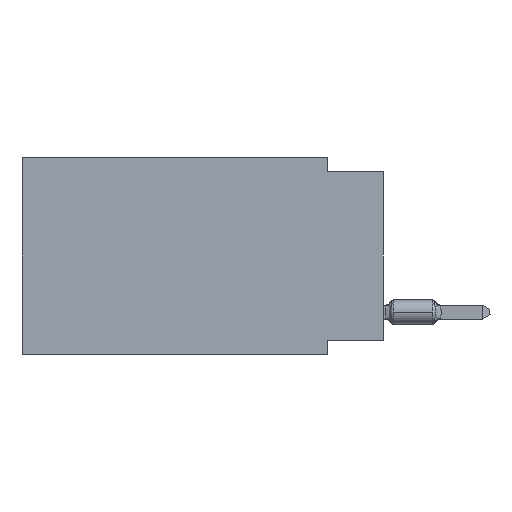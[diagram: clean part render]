
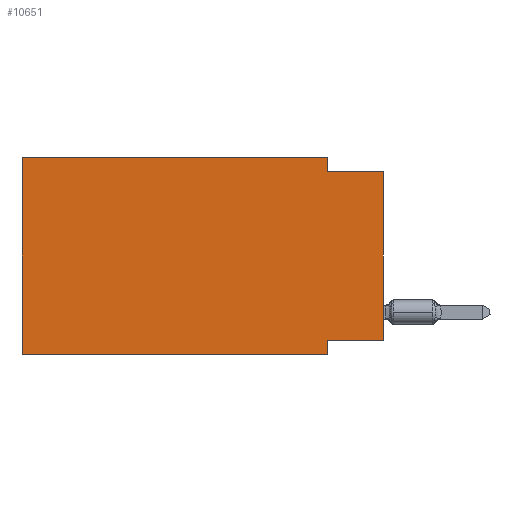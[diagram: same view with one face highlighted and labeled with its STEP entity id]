
A CAD part, left-side view. The second image highlights one B-rep face of the part: STEP entity #10651.
In plain terms, the highlighted planar face has unit normal (-1, 0, 0).
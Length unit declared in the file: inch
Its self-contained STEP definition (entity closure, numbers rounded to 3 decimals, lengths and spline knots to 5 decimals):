
#71 = VERTEX_POINT ( 'NONE', #4853 ) ;
#586 = VECTOR ( 'NONE', #7887, 39.37008 ) ;
#1035 = CARTESIAN_POINT ( 'NONE',  ( 0., 0., -0.025 ) ) ;
#1138 = VERTEX_POINT ( 'NONE', #14995 ) ;
#1370 = CARTESIAN_POINT ( 'NONE',  ( 0., 0.1, 0. ) ) ;
#1806 = LINE ( 'NONE', #6784, #7038 ) ;
#2073 = CARTESIAN_POINT ( 'NONE',  ( 0., 0., -0.325 ) ) ;
#2332 = CARTESIAN_POINT ( 'NONE',  ( 0., 0., 0. ) ) ;
#2393 = EDGE_CURVE ( 'NONE', #21580, #5204, #20155, .T. ) ;
#3198 = DIRECTION ( 'NONE',  ( 0., 0., -1. ) ) ;
#3773 = EDGE_LOOP ( 'NONE', ( #19470, #11132, #13963, #9775, #19159, #15180, #14685, #8173 ) ) ;
#4623 = LINE ( 'NONE', #13487, #4874 ) ;
#4830 = EDGE_CURVE ( 'NONE', #1138, #12046, #4623, .T. ) ;
#4840 = LINE ( 'NONE', #1035, #19109 ) ;
#4853 = CARTESIAN_POINT ( 'NONE',  ( 0., 0.1, -0.325 ) ) ;
#4874 = VECTOR ( 'NONE', #21982, 39.37008 ) ;
#5204 = VERTEX_POINT ( 'NONE', #16688 ) ;
#5229 = PLANE ( 'NONE',  #11575 ) ;
#5503 = EDGE_CURVE ( 'NONE', #12060, #8527, #16630, .T. ) ;
#6114 = LINE ( 'NONE', #13120, #12769 ) ;
#6492 = EDGE_CURVE ( 'NONE', #1138, #12060, #6114, .T. ) ;
#6784 = CARTESIAN_POINT ( 'NONE',  ( 0., 0.1, 0. ) ) ;
#7038 = VECTOR ( 'NONE', #3198, 39.37008 ) ;
#7044 = LINE ( 'NONE', #2073, #11892 ) ;
#7887 = DIRECTION ( 'NONE',  ( 0., -1., 0. ) ) ;
#7983 = DIRECTION ( 'NONE',  ( 0., 0., 1. ) ) ;
#8173 = ORIENTED_EDGE ( 'NONE', *, *, #16209, .F. ) ;
#8329 = CARTESIAN_POINT ( 'NONE',  ( 0., 0.1, -0.025 ) ) ;
#8519 = EDGE_CURVE ( 'NONE', #18264, #5204, #4840, .T. ) ;
#8527 = VERTEX_POINT ( 'NONE', #1370 ) ;
#8571 = DIRECTION ( 'NONE',  ( 0., 0., -1. ) ) ;
#8998 = DIRECTION ( 'NONE',  ( 0., 1., 0. ) ) ;
#9085 = CARTESIAN_POINT ( 'NONE',  ( 0., 0., -0.325 ) ) ;
#9775 = ORIENTED_EDGE ( 'NONE', *, *, #5503, .F. ) ;
#10627 = LINE ( 'NONE', #16151, #10978 ) ;
#10651 = ADVANCED_FACE ( 'NONE', ( #13857 ), #5229, .F. ) ;
#10971 = DIRECTION ( 'NONE',  ( 0., 0., -1. ) ) ;
#10978 = VECTOR ( 'NONE', #10971, 39.37008 ) ;
#11132 = ORIENTED_EDGE ( 'NONE', *, *, #8519, .F. ) ;
#11398 = DIRECTION ( 'NONE',  ( 0., 0., 1. ) ) ;
#11575 = AXIS2_PLACEMENT_3D ( 'NONE', #12255, #20971, #8571 ) ;
#11892 = VECTOR ( 'NONE', #8998, 39.37008 ) ;
#12046 = VERTEX_POINT ( 'NONE', #18453 ) ;
#12060 = VERTEX_POINT ( 'NONE', #16734 ) ;
#12255 = CARTESIAN_POINT ( 'NONE',  ( 0., 0.645, 0. ) ) ;
#12769 = VECTOR ( 'NONE', #11398, 39.37008 ) ;
#13120 = CARTESIAN_POINT ( 'NONE',  ( 0., 0.645, 0. ) ) ;
#13487 = CARTESIAN_POINT ( 'NONE',  ( 0., 0.645, -0.35 ) ) ;
#13857 = FACE_OUTER_BOUND ( 'NONE', #3773, .T. ) ;
#13963 = ORIENTED_EDGE ( 'NONE', *, *, #14209, .F. ) ;
#14209 = EDGE_CURVE ( 'NONE', #8527, #18264, #1806, .T. ) ;
#14685 = ORIENTED_EDGE ( 'NONE', *, *, #19703, .F. ) ;
#14995 = CARTESIAN_POINT ( 'NONE',  ( 0., 0.645, -0.35 ) ) ;
#15180 = ORIENTED_EDGE ( 'NONE', *, *, #4830, .T. ) ;
#16151 = CARTESIAN_POINT ( 'NONE',  ( 0., 0.1, -0.35 ) ) ;
#16209 = EDGE_CURVE ( 'NONE', #21580, #71, #7044, .T. ) ;
#16630 = LINE ( 'NONE', #21781, #586 ) ;
#16688 = CARTESIAN_POINT ( 'NONE',  ( 0., 0., -0.025 ) ) ;
#16734 = CARTESIAN_POINT ( 'NONE',  ( 0., 0.645, 0. ) ) ;
#18264 = VERTEX_POINT ( 'NONE', #8329 ) ;
#18453 = CARTESIAN_POINT ( 'NONE',  ( 0., 0.1, -0.35 ) ) ;
#19109 = VECTOR ( 'NONE', #21981, 39.37008 ) ;
#19159 = ORIENTED_EDGE ( 'NONE', *, *, #6492, .F. ) ;
#19212 = VECTOR ( 'NONE', #7983, 39.37008 ) ;
#19470 = ORIENTED_EDGE ( 'NONE', *, *, #2393, .T. ) ;
#19703 = EDGE_CURVE ( 'NONE', #71, #12046, #10627, .T. ) ;
#20155 = LINE ( 'NONE', #2332, #19212 ) ;
#20971 = DIRECTION ( 'NONE',  ( 1., 0., 0. ) ) ;
#21580 = VERTEX_POINT ( 'NONE', #9085 ) ;
#21781 = CARTESIAN_POINT ( 'NONE',  ( 0., 0.645, 0. ) ) ;
#21981 = DIRECTION ( 'NONE',  ( 0., -1., 0. ) ) ;
#21982 = DIRECTION ( 'NONE',  ( 0., -1., 0. ) ) ;
